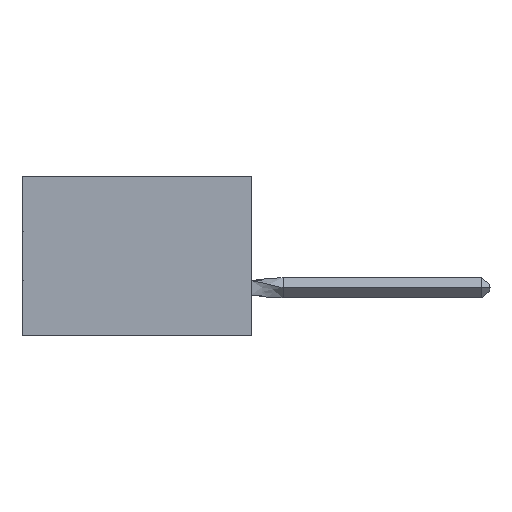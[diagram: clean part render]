
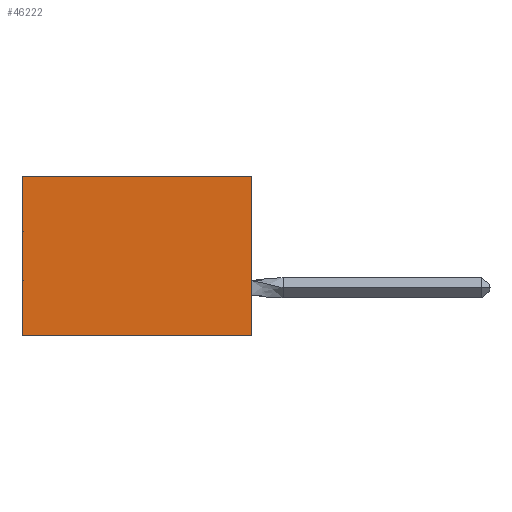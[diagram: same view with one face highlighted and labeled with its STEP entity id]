
A CAD part, left-side view. The second image highlights one B-rep face of the part: STEP entity #46222.
In plain terms, the highlighted planar face has unit normal (-1, 0, 0).
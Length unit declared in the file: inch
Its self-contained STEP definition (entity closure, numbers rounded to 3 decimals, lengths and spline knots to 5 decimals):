
#1534 = VERTEX_POINT ( 'NONE', #47825 ) ;
#3535 = LINE ( 'NONE', #39731, #6639 ) ;
#4834 = CARTESIAN_POINT ( 'NONE',  ( 0.305, 0., 0. ) ) ;
#5272 = CARTESIAN_POINT ( 'NONE',  ( 0.305, 0., -0.5 ) ) ;
#6551 = EDGE_LOOP ( 'NONE', ( #17884, #11014, #24037, #17253 ) ) ;
#6639 = VECTOR ( 'NONE', #31182, 39.37008 ) ;
#7952 = LINE ( 'NONE', #47522, #43357 ) ;
#8377 = CARTESIAN_POINT ( 'NONE',  ( 0.305, 0., -0.5 ) ) ;
#11014 = ORIENTED_EDGE ( 'NONE', *, *, #25111, .F. ) ;
#11359 = VECTOR ( 'NONE', #15140, 39.37008 ) ;
#13121 = FACE_OUTER_BOUND ( 'NONE', #6551, .T. ) ;
#13304 = EDGE_CURVE ( 'NONE', #13922, #21799, #7952, .T. ) ;
#13405 = DIRECTION ( 'NONE',  ( 1., 0., 0. ) ) ;
#13922 = VERTEX_POINT ( 'NONE', #4834 ) ;
#15140 = DIRECTION ( 'NONE',  ( 0., 0., -1. ) ) ;
#15758 = LINE ( 'NONE', #8377, #40665 ) ;
#16765 = PLANE ( 'NONE',  #22931 ) ;
#17253 = ORIENTED_EDGE ( 'NONE', *, *, #13304, .T. ) ;
#17884 = ORIENTED_EDGE ( 'NONE', *, *, #38596, .T. ) ;
#19696 = EDGE_CURVE ( 'NONE', #13922, #48173, #15758, .T. ) ;
#19978 = DIRECTION ( 'NONE',  ( 0., 0., -1. ) ) ;
#21799 = VERTEX_POINT ( 'NONE', #48154 ) ;
#22931 = AXIS2_PLACEMENT_3D ( 'NONE', #5272, #13405, #28742 ) ;
#24037 = ORIENTED_EDGE ( 'NONE', *, *, #19696, .F. ) ;
#25111 = EDGE_CURVE ( 'NONE', #48173, #1534, #3535, .T. ) ;
#28742 = DIRECTION ( 'NONE',  ( 0., 0., -1. ) ) ;
#31182 = DIRECTION ( 'NONE',  ( 0., 1., 0. ) ) ;
#35542 = DIRECTION ( 'NONE',  ( 0., 1., 0. ) ) ;
#36063 = CARTESIAN_POINT ( 'NONE',  ( 0.305, 0., -0.5 ) ) ;
#38596 = EDGE_CURVE ( 'NONE', #21799, #1534, #46805, .T. ) ;
#39731 = CARTESIAN_POINT ( 'NONE',  ( 0.305, 0., -0.5 ) ) ;
#40665 = VECTOR ( 'NONE', #19978, 39.37008 ) ;
#43357 = VECTOR ( 'NONE', #35542, 39.37008 ) ;
#46222 = ADVANCED_FACE ( 'NONE', ( #13121 ), #16765, .F. ) ;
#46805 = LINE ( 'NONE', #50813, #11359 ) ;
#47522 = CARTESIAN_POINT ( 'NONE',  ( 0.305, 0., 0. ) ) ;
#47825 = CARTESIAN_POINT ( 'NONE',  ( 0.305, 0.72, -0.5 ) ) ;
#48154 = CARTESIAN_POINT ( 'NONE',  ( 0.305, 0.72, 0. ) ) ;
#48173 = VERTEX_POINT ( 'NONE', #36063 ) ;
#50813 = CARTESIAN_POINT ( 'NONE',  ( 0.305, 0.72, -0.5 ) ) ;
